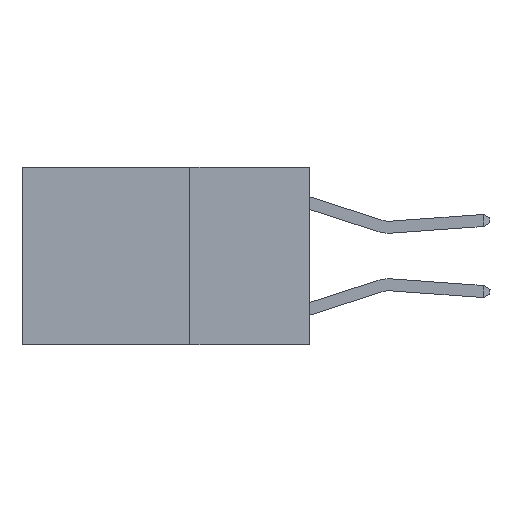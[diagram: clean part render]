
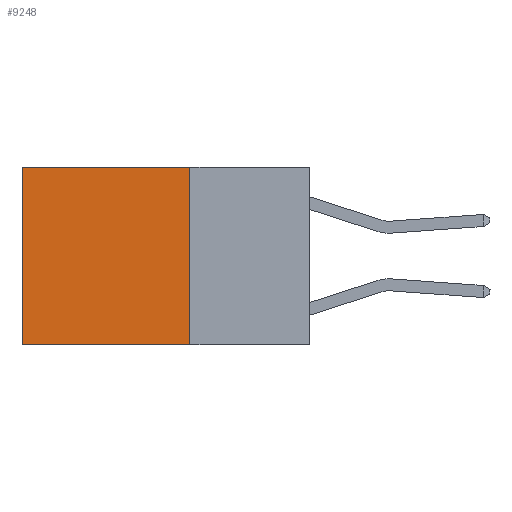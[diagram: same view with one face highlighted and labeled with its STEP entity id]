
A CAD part, left-side view. The second image highlights one B-rep face of the part: STEP entity #9248.
In plain terms, the highlighted planar face has unit normal (-1, 0, 0).
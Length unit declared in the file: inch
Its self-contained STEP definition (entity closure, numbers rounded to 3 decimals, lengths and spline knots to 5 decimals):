
#886 = VERTEX_POINT ( 'NONE', #8875 ) ;
#1328 = LINE ( 'NONE', #29531, #26220 ) ;
#2302 = VECTOR ( 'NONE', #17857, 39.37008 ) ;
#2770 = EDGE_CURVE ( 'NONE', #886, #3146, #6276, .T. ) ;
#3000 = CARTESIAN_POINT ( 'NONE',  ( 0.2625, 0.6, 0. ) ) ;
#3146 = VERTEX_POINT ( 'NONE', #3000 ) ;
#3379 = VERTEX_POINT ( 'NONE', #23130 ) ;
#5200 = EDGE_CURVE ( 'NONE', #886, #3379, #16749, .T. ) ;
#5247 = EDGE_CURVE ( 'NONE', #3146, #5450, #28301, .T. ) ;
#5450 = VERTEX_POINT ( 'NONE', #25723 ) ;
#5560 = CARTESIAN_POINT ( 'NONE',  ( 0.2625, 0.25, 0. ) ) ;
#6255 = AXIS2_PLACEMENT_3D ( 'NONE', #27941, #13682, #30312 ) ;
#6276 = LINE ( 'NONE', #25656, #13538 ) ;
#7168 = ORIENTED_EDGE ( 'NONE', *, *, #2770, .T. ) ;
#8282 = EDGE_CURVE ( 'NONE', #3379, #5450, #1328, .T. ) ;
#8875 = CARTESIAN_POINT ( 'NONE',  ( 0.2625, 0.25, 0. ) ) ;
#9248 = ADVANCED_FACE ( 'NONE', ( #28094 ), #27837, .F. ) ;
#10432 = DIRECTION ( 'NONE',  ( 0., 1., 0. ) ) ;
#13538 = VECTOR ( 'NONE', #18617, 39.37008 ) ;
#13682 = DIRECTION ( 'NONE',  ( 1., 0., 0. ) ) ;
#16749 = LINE ( 'NONE', #5560, #23085 ) ;
#16812 = ORIENTED_EDGE ( 'NONE', *, *, #5247, .T. ) ;
#17641 = DIRECTION ( 'NONE',  ( 0., 0., -1. ) ) ;
#17739 = CARTESIAN_POINT ( 'NONE',  ( 0.2625, 0.6, 0. ) ) ;
#17857 = DIRECTION ( 'NONE',  ( 0., 0., -1. ) ) ;
#18617 = DIRECTION ( 'NONE',  ( 0., 1., 0. ) ) ;
#18627 = ORIENTED_EDGE ( 'NONE', *, *, #8282, .F. ) ;
#23085 = VECTOR ( 'NONE', #17641, 39.37008 ) ;
#23130 = CARTESIAN_POINT ( 'NONE',  ( 0.2625, 0.25, -0.37 ) ) ;
#24656 = ORIENTED_EDGE ( 'NONE', *, *, #5200, .F. ) ;
#25656 = CARTESIAN_POINT ( 'NONE',  ( 0.2625, 0.25, 0. ) ) ;
#25723 = CARTESIAN_POINT ( 'NONE',  ( 0.2625, 0.6, -0.37 ) ) ;
#26220 = VECTOR ( 'NONE', #10432, 39.37008 ) ;
#27837 = PLANE ( 'NONE',  #6255 ) ;
#27941 = CARTESIAN_POINT ( 'NONE',  ( 0.2625, 0.25, 0. ) ) ;
#28051 = EDGE_LOOP ( 'NONE', ( #16812, #18627, #24656, #7168 ) ) ;
#28094 = FACE_OUTER_BOUND ( 'NONE', #28051, .T. ) ;
#28301 = LINE ( 'NONE', #17739, #2302 ) ;
#29531 = CARTESIAN_POINT ( 'NONE',  ( 0.2625, 0.25, -0.37 ) ) ;
#30312 = DIRECTION ( 'NONE',  ( 0., 0., -1. ) ) ;
